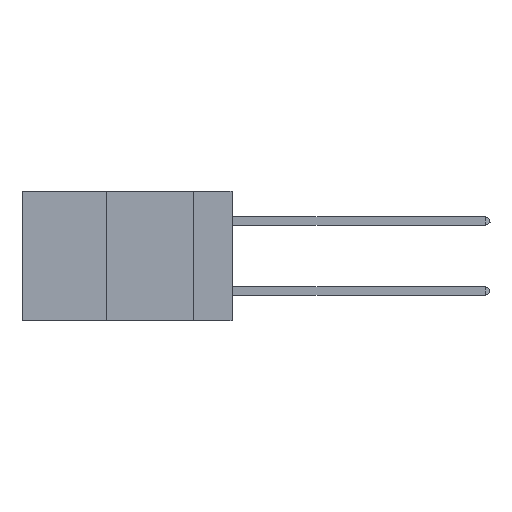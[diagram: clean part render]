
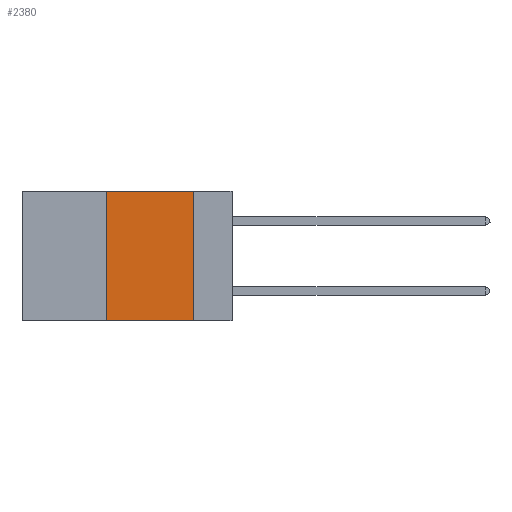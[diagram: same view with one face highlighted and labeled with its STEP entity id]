
A CAD part, left-side view. The second image highlights one B-rep face of the part: STEP entity #2380.
In plain terms, the highlighted planar face has unit normal (-1, 0, 0).
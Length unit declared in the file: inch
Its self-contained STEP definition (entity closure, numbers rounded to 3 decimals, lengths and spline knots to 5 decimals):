
#601 = DIRECTION ( 'NONE',  ( 0., -1., 0. ) ) ;
#892 = CARTESIAN_POINT ( 'NONE',  ( 0., 0.36, 0. ) ) ;
#1417 = VERTEX_POINT ( 'NONE', #9383 ) ;
#2127 = VECTOR ( 'NONE', #11305, 39.37008 ) ;
#2330 = VERTEX_POINT ( 'NONE', #5995 ) ;
#2380 = ADVANCED_FACE ( 'NONE', ( #11950 ), #11125, .F. ) ;
#2417 = VECTOR ( 'NONE', #5206, 39.37008 ) ;
#2455 = ORIENTED_EDGE ( 'NONE', *, *, #14568, .F. ) ;
#3074 = LINE ( 'NONE', #10179, #2127 ) ;
#3117 = ORIENTED_EDGE ( 'NONE', *, *, #4184, .F. ) ;
#3186 = AXIS2_PLACEMENT_3D ( 'NONE', #4282, #14455, #4204 ) ;
#4184 = EDGE_CURVE ( 'NONE', #2330, #13881, #3074, .T. ) ;
#4204 = DIRECTION ( 'NONE',  ( 0., 0., -1. ) ) ;
#4282 = CARTESIAN_POINT ( 'NONE',  ( 0., 0.6, 0. ) ) ;
#5186 = CARTESIAN_POINT ( 'NONE',  ( 0., 0.6, 0. ) ) ;
#5206 = DIRECTION ( 'NONE',  ( 0., 0., 1. ) ) ;
#5593 = CARTESIAN_POINT ( 'NONE',  ( 0., 0.11, -0.37 ) ) ;
#5995 = CARTESIAN_POINT ( 'NONE',  ( 0., 0.11, 0. ) ) ;
#6037 = VERTEX_POINT ( 'NONE', #8449 ) ;
#6061 = EDGE_CURVE ( 'NONE', #1417, #2330, #6234, .T. ) ;
#6234 = LINE ( 'NONE', #5186, #14614 ) ;
#6250 = LINE ( 'NONE', #892, #2417 ) ;
#6345 = VECTOR ( 'NONE', #601, 39.37008 ) ;
#6375 = DIRECTION ( 'NONE',  ( 0., -1., 0. ) ) ;
#7548 = EDGE_CURVE ( 'NONE', #6037, #13881, #9874, .T. ) ;
#7895 = CARTESIAN_POINT ( 'NONE',  ( 0., 0.6, -0.37 ) ) ;
#8137 = ORIENTED_EDGE ( 'NONE', *, *, #7548, .T. ) ;
#8449 = CARTESIAN_POINT ( 'NONE',  ( 0., 0.36, -0.37 ) ) ;
#9383 = CARTESIAN_POINT ( 'NONE',  ( 0., 0.36, 0. ) ) ;
#9874 = LINE ( 'NONE', #7895, #6345 ) ;
#10041 = EDGE_LOOP ( 'NONE', ( #3117, #11603, #2455, #8137 ) ) ;
#10179 = CARTESIAN_POINT ( 'NONE',  ( 0., 0.11, 0. ) ) ;
#11125 = PLANE ( 'NONE',  #3186 ) ;
#11305 = DIRECTION ( 'NONE',  ( 0., 0., -1. ) ) ;
#11603 = ORIENTED_EDGE ( 'NONE', *, *, #6061, .F. ) ;
#11950 = FACE_OUTER_BOUND ( 'NONE', #10041, .T. ) ;
#13881 = VERTEX_POINT ( 'NONE', #5593 ) ;
#14455 = DIRECTION ( 'NONE',  ( 1., 0., 0. ) ) ;
#14568 = EDGE_CURVE ( 'NONE', #6037, #1417, #6250, .T. ) ;
#14614 = VECTOR ( 'NONE', #6375, 39.37008 ) ;
